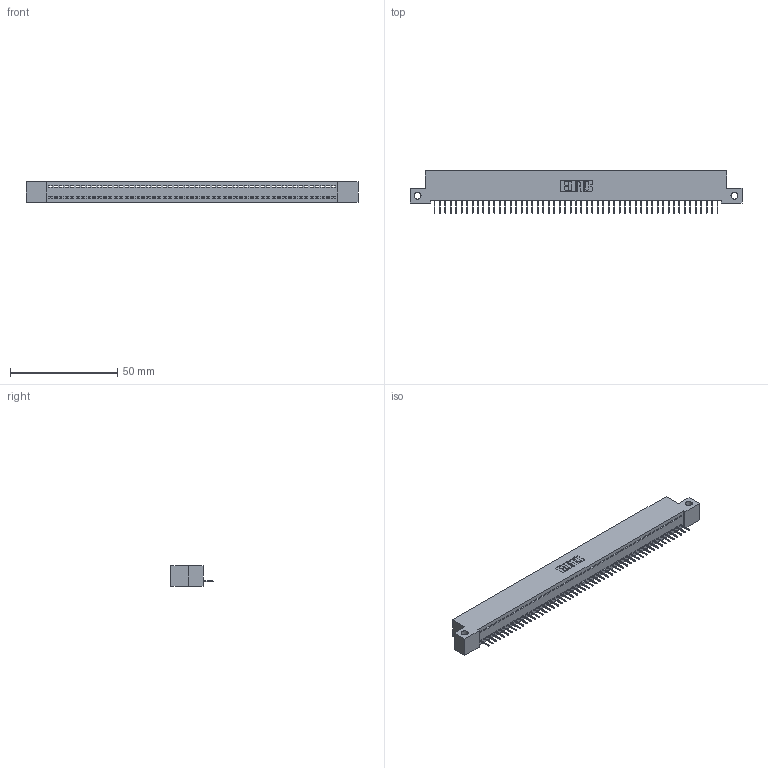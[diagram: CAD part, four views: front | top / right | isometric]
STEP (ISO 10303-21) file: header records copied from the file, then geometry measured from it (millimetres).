
FILE_DESCRIPTION (( 'STEP AP203' ), '1' );
FILE_NAME ('392-053-524-112.STEP', '2018-08-17T07:16:27', ( '' ), ( '' ), 'SwSTEP 2.0', 'SolidWorks 2016', '' );
FILE_SCHEMA (( 'CONFIG_CONTROL_DESIGN' ));
Length unit declared in the file: inch
Products named in the file (3): 345-292-001_345-293-124; 392-053-524-112; 342 Part_Side Mount
Assembly tree (54 placements, depth 2):
  392-053-524-112
    342 Part_Side Mount
    345-292-001_345-293-124  x53
Bounding box: 154.94 x 19.69 x 9.4 mm (x, y, z)
Volume: 13342.4 mm3; surface area: 18984.6 mm2
Topology: 54 solids, 54 shells, 3396 faces, 9839 edges, 6346 vertices
Faces by surface type: plane 2610, cylinder 786
Entity records: 30923 total; most frequent: CARTESIAN_POINT 5337, ORIENTED_EDGE 5326, DIRECTION 4481, EDGE_CURVE 2663, LINE 2539, VECTOR 2539, VERTEX_POINT 1770, AXIS2_PLACEMENT_3D 971
